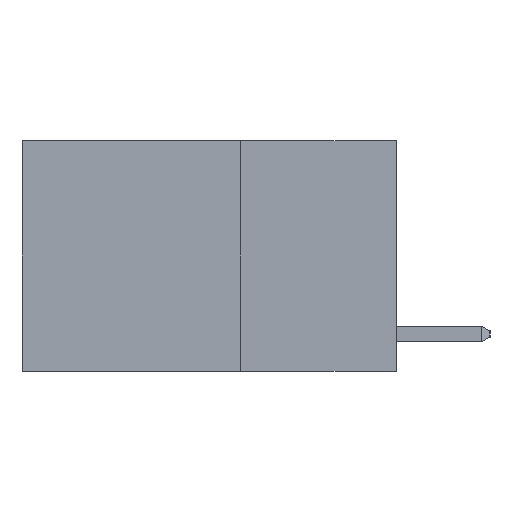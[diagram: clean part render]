
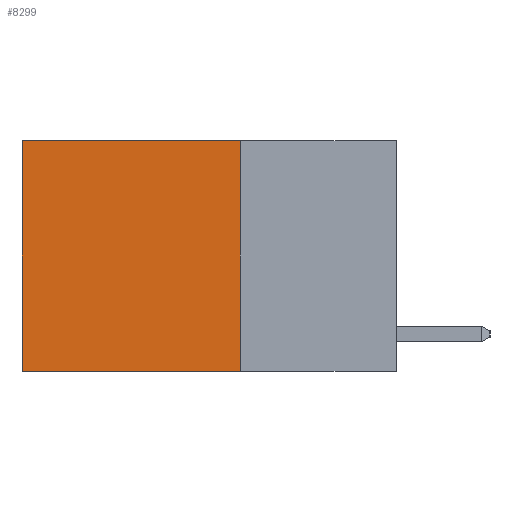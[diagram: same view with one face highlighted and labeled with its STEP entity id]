
A CAD part, left-side view. The second image highlights one B-rep face of the part: STEP entity #8299.
In plain terms, the highlighted planar face has unit normal (-1, 0, 0).
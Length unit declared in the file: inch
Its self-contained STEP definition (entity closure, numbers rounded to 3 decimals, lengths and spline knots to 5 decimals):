
#239 = CARTESIAN_POINT ( 'NONE',  ( 0.2625, 0.6, -0.37 ) ) ;
#847 = VERTEX_POINT ( 'NONE', #7021 ) ;
#1237 = PLANE ( 'NONE',  #7900 ) ;
#1238 = CARTESIAN_POINT ( 'NONE',  ( 0.2625, 0.25, -0.37 ) ) ;
#1490 = VERTEX_POINT ( 'NONE', #1238 ) ;
#1687 = VECTOR ( 'NONE', #8849, 39.37008 ) ;
#1731 = ORIENTED_EDGE ( 'NONE', *, *, #2000, .T. ) ;
#2000 = EDGE_CURVE ( 'NONE', #4921, #847, #5673, .T. ) ;
#2007 = CARTESIAN_POINT ( 'NONE',  ( 0.2625, 0.25, 0. ) ) ;
#2225 = VERTEX_POINT ( 'NONE', #239 ) ;
#2304 = FACE_OUTER_BOUND ( 'NONE', #4334, .T. ) ;
#2450 = EDGE_CURVE ( 'NONE', #1490, #2225, #5192, .T. ) ;
#2827 = DIRECTION ( 'NONE',  ( 0., 0., -1. ) ) ;
#3005 = CARTESIAN_POINT ( 'NONE',  ( 0.2625, 0.25, 0. ) ) ;
#3494 = DIRECTION ( 'NONE',  ( 1., 0., 0. ) ) ;
#3736 = DIRECTION ( 'NONE',  ( 0., 0., -1. ) ) ;
#4334 = EDGE_LOOP ( 'NONE', ( #8316, #7689, #5944, #1731 ) ) ;
#4921 = VERTEX_POINT ( 'NONE', #5784 ) ;
#5192 = LINE ( 'NONE', #8093, #8993 ) ;
#5673 = LINE ( 'NONE', #6210, #1687 ) ;
#5784 = CARTESIAN_POINT ( 'NONE',  ( 0.2625, 0.25, 0. ) ) ;
#5802 = EDGE_CURVE ( 'NONE', #847, #2225, #7666, .T. ) ;
#5822 = DIRECTION ( 'NONE',  ( 0., 1., 0. ) ) ;
#5944 = ORIENTED_EDGE ( 'NONE', *, *, #8499, .F. ) ;
#6210 = CARTESIAN_POINT ( 'NONE',  ( 0.2625, 0.25, 0. ) ) ;
#6684 = VECTOR ( 'NONE', #3736, 39.37008 ) ;
#7021 = CARTESIAN_POINT ( 'NONE',  ( 0.2625, 0.6, 0. ) ) ;
#7426 = VECTOR ( 'NONE', #2827, 39.37008 ) ;
#7666 = LINE ( 'NONE', #8125, #7426 ) ;
#7689 = ORIENTED_EDGE ( 'NONE', *, *, #2450, .F. ) ;
#7900 = AXIS2_PLACEMENT_3D ( 'NONE', #2007, #3494, #8780 ) ;
#8093 = CARTESIAN_POINT ( 'NONE',  ( 0.2625, 0.25, -0.37 ) ) ;
#8125 = CARTESIAN_POINT ( 'NONE',  ( 0.2625, 0.6, 0. ) ) ;
#8204 = LINE ( 'NONE', #3005, #6684 ) ;
#8299 = ADVANCED_FACE ( 'NONE', ( #2304 ), #1237, .F. ) ;
#8316 = ORIENTED_EDGE ( 'NONE', *, *, #5802, .T. ) ;
#8499 = EDGE_CURVE ( 'NONE', #4921, #1490, #8204, .T. ) ;
#8780 = DIRECTION ( 'NONE',  ( 0., 0., -1. ) ) ;
#8849 = DIRECTION ( 'NONE',  ( 0., 1., 0. ) ) ;
#8993 = VECTOR ( 'NONE', #5822, 39.37008 ) ;
